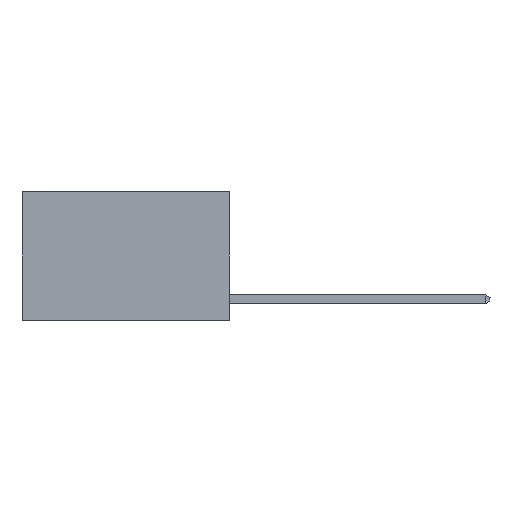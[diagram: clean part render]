
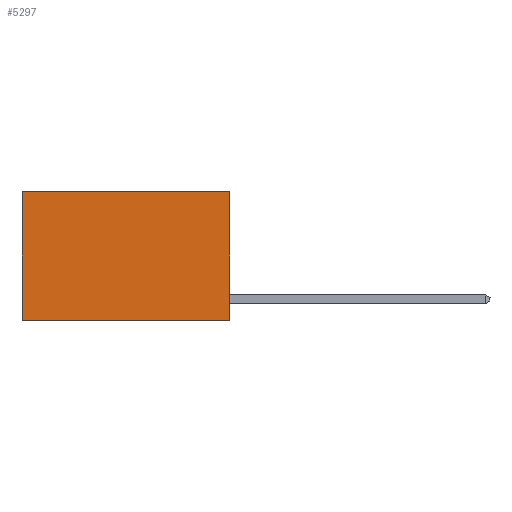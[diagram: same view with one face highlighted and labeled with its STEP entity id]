
A CAD part, left-side view. The second image highlights one B-rep face of the part: STEP entity #5297.
In plain terms, the highlighted planar face has unit normal (-1, 0, 0).
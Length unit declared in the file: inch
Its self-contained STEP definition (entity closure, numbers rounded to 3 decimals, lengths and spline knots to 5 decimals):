
#155 = EDGE_CURVE ( 'NONE', #487, #8372, #19031, .T. ) ;
#487 = VERTEX_POINT ( 'NONE', #8835 ) ;
#660 = EDGE_CURVE ( 'NONE', #487, #16871, #20211, .T. ) ;
#1831 = CARTESIAN_POINT ( 'NONE',  ( 0.2625, 0.6, 0. ) ) ;
#2460 = CARTESIAN_POINT ( 'NONE',  ( 0.2625, 0.6, -0.37 ) ) ;
#2972 = CARTESIAN_POINT ( 'NONE',  ( 0.2625, 0., 0. ) ) ;
#3116 = LINE ( 'NONE', #12545, #3283 ) ;
#3283 = VECTOR ( 'NONE', #12788, 39.37008 ) ;
#4846 = CARTESIAN_POINT ( 'NONE',  ( 0.2625, 0., 0. ) ) ;
#5297 = ADVANCED_FACE ( 'NONE', ( #16009 ), #12610, .F. ) ;
#5304 = ORIENTED_EDGE ( 'NONE', *, *, #660, .T. ) ;
#6143 = EDGE_CURVE ( 'NONE', #8372, #12497, #11010, .T. ) ;
#7496 = CARTESIAN_POINT ( 'NONE',  ( 0.2625, 0., -0.37 ) ) ;
#8372 = VERTEX_POINT ( 'NONE', #9325 ) ;
#8835 = CARTESIAN_POINT ( 'NONE',  ( 0.2625, 0., 0. ) ) ;
#9325 = CARTESIAN_POINT ( 'NONE',  ( 0.2625, 0., -0.37 ) ) ;
#10640 = DIRECTION ( 'NONE',  ( 0., 1., 0. ) ) ;
#11010 = LINE ( 'NONE', #7496, #21523 ) ;
#11235 = ORIENTED_EDGE ( 'NONE', *, *, #6143, .F. ) ;
#12497 = VERTEX_POINT ( 'NONE', #2460 ) ;
#12545 = CARTESIAN_POINT ( 'NONE',  ( 0.2625, 0.6, 0. ) ) ;
#12610 = PLANE ( 'NONE',  #15050 ) ;
#12755 = DIRECTION ( 'NONE',  ( 0., 1., 0. ) ) ;
#12788 = DIRECTION ( 'NONE',  ( 0., 0., -1. ) ) ;
#13303 = ORIENTED_EDGE ( 'NONE', *, *, #155, .F. ) ;
#13480 = EDGE_CURVE ( 'NONE', #16871, #12497, #3116, .T. ) ;
#14422 = ORIENTED_EDGE ( 'NONE', *, *, #13480, .T. ) ;
#14571 = EDGE_LOOP ( 'NONE', ( #14422, #11235, #13303, #5304 ) ) ;
#15050 = AXIS2_PLACEMENT_3D ( 'NONE', #4846, #20296, #17905 ) ;
#15655 = VECTOR ( 'NONE', #22676, 39.37008 ) ;
#16009 = FACE_OUTER_BOUND ( 'NONE', #14571, .T. ) ;
#16871 = VERTEX_POINT ( 'NONE', #1831 ) ;
#17201 = VECTOR ( 'NONE', #10640, 39.37008 ) ;
#17905 = DIRECTION ( 'NONE',  ( 0., 0., -1. ) ) ;
#19031 = LINE ( 'NONE', #21287, #15655 ) ;
#20211 = LINE ( 'NONE', #2972, #17201 ) ;
#20296 = DIRECTION ( 'NONE',  ( 1., 0., 0. ) ) ;
#21287 = CARTESIAN_POINT ( 'NONE',  ( 0.2625, 0., 0. ) ) ;
#21523 = VECTOR ( 'NONE', #12755, 39.37008 ) ;
#22676 = DIRECTION ( 'NONE',  ( 0., 0., -1. ) ) ;
